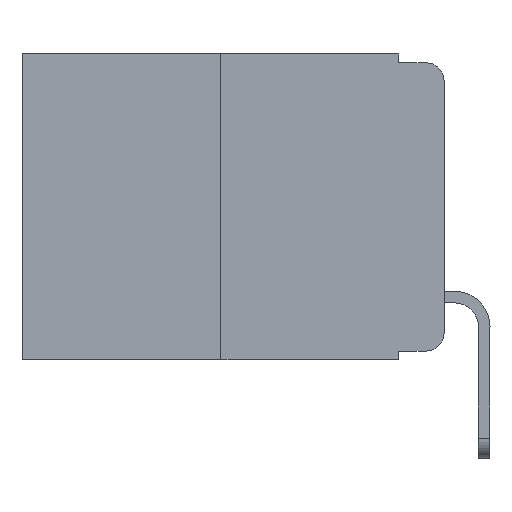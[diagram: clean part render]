
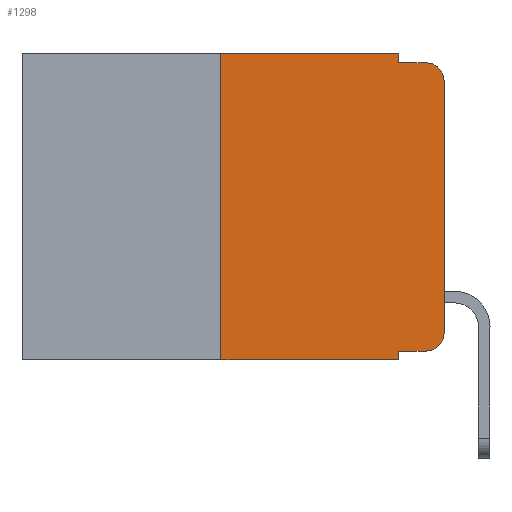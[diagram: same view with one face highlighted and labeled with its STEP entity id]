
A CAD part, left-side view. The second image highlights one B-rep face of the part: STEP entity #1298.
In plain terms, the highlighted planar face has unit normal (-1, 0, 0).
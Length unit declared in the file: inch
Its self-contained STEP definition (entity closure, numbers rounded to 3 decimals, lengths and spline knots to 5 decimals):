
#340 = VECTOR ( 'NONE', #1689, 39.37008 ) ;
#1086 = LINE ( 'NONE', #12152, #5563 ) ;
#1298 = ADVANCED_FACE ( 'NONE', ( #9779 ), #1872, .F. ) ;
#1528 = DIRECTION ( 'NONE',  ( -1., 0., 0. ) ) ;
#1554 = EDGE_CURVE ( 'NONE', #5342, #3291, #9195, .T. ) ;
#1689 = DIRECTION ( 'NONE',  ( 0., 0., 1. ) ) ;
#1758 = CARTESIAN_POINT ( 'NONE',  ( 0., 0.473, 0. ) ) ;
#1872 = PLANE ( 'NONE',  #3984 ) ;
#2071 = CARTESIAN_POINT ( 'NONE',  ( 0., 0., -0.03 ) ) ;
#2209 = LINE ( 'NONE', #12271, #6872 ) ;
#2765 = VERTEX_POINT ( 'NONE', #12022 ) ;
#2840 = VECTOR ( 'NONE', #3044, 39.37008 ) ;
#2890 = DIRECTION ( 'NONE',  ( 0., -1., 0. ) ) ;
#3044 = DIRECTION ( 'NONE',  ( 0., -1., 0. ) ) ;
#3227 = ORIENTED_EDGE ( 'NONE', *, *, #10108, .T. ) ;
#3291 = VERTEX_POINT ( 'NONE', #4524 ) ;
#3742 = DIRECTION ( 'NONE',  ( 0., 0., -1. ) ) ;
#3973 = ORIENTED_EDGE ( 'NONE', *, *, #14810, .F. ) ;
#3984 = AXIS2_PLACEMENT_3D ( 'NONE', #5562, #14246, #12817 ) ;
#4219 = EDGE_CURVE ( 'NONE', #8052, #2765, #6016, .T. ) ;
#4456 = EDGE_CURVE ( 'NONE', #11386, #15500, #11391, .T. ) ;
#4524 = CARTESIAN_POINT ( 'NONE',  ( 0., 0., -0.313 ) ) ;
#4906 = DIRECTION ( 'NONE',  ( 0., -1., 0. ) ) ;
#5342 = VERTEX_POINT ( 'NONE', #9818 ) ;
#5562 = CARTESIAN_POINT ( 'NONE',  ( 0., 0.473, 0. ) ) ;
#5563 = VECTOR ( 'NONE', #10189, 39.37008 ) ;
#5622 = EDGE_CURVE ( 'NONE', #15500, #10020, #9814, .T. ) ;
#6016 = CIRCLE ( 'NONE', #8974, 0.02 ) ;
#6192 = LINE ( 'NONE', #9088, #340 ) ;
#6570 = CARTESIAN_POINT ( 'NONE',  ( 0., 0.02, -0.03 ) ) ;
#6620 = ORIENTED_EDGE ( 'NONE', *, *, #5622, .F. ) ;
#6689 = AXIS2_PLACEMENT_3D ( 'NONE', #9867, #15855, #8411 ) ;
#6872 = VECTOR ( 'NONE', #4906, 39.37008 ) ;
#7347 = LINE ( 'NONE', #8785, #8878 ) ;
#7410 = CARTESIAN_POINT ( 'NONE',  ( 0., 0.25, 0. ) ) ;
#7444 = EDGE_CURVE ( 'NONE', #13667, #2765, #2209, .T. ) ;
#7505 = CARTESIAN_POINT ( 'NONE',  ( 0., 0.473, -0.343 ) ) ;
#7801 = DIRECTION ( 'NONE',  ( 0., 0., -1. ) ) ;
#7888 = EDGE_LOOP ( 'NONE', ( #14979, #8328, #7933, #9356, #6620, #11798, #13872, #3973, #3227, #8174 ) ) ;
#7933 = ORIENTED_EDGE ( 'NONE', *, *, #7444, .F. ) ;
#8052 = VERTEX_POINT ( 'NONE', #2071 ) ;
#8134 = CARTESIAN_POINT ( 'NONE',  ( 0., 0.25, 0. ) ) ;
#8174 = ORIENTED_EDGE ( 'NONE', *, *, #1554, .T. ) ;
#8244 = VECTOR ( 'NONE', #3742, 39.37008 ) ;
#8328 = ORIENTED_EDGE ( 'NONE', *, *, #4219, .T. ) ;
#8411 = DIRECTION ( 'NONE',  ( 0., 0., -1. ) ) ;
#8655 = VECTOR ( 'NONE', #11267, 39.37008 ) ;
#8785 = CARTESIAN_POINT ( 'NONE',  ( 0., 0.051, -0.333 ) ) ;
#8795 = CARTESIAN_POINT ( 'NONE',  ( 0., 0.051, -0.01 ) ) ;
#8878 = VECTOR ( 'NONE', #2890, 39.37008 ) ;
#8974 = AXIS2_PLACEMENT_3D ( 'NONE', #6570, #1528, #7801 ) ;
#9088 = CARTESIAN_POINT ( 'NONE',  ( 0., 0., 0. ) ) ;
#9195 = CIRCLE ( 'NONE', #6689, 0.02 ) ;
#9276 = VERTEX_POINT ( 'NONE', #11964 ) ;
#9356 = ORIENTED_EDGE ( 'NONE', *, *, #14271, .F. ) ;
#9587 = DIRECTION ( 'NONE',  ( 0., 0., 1. ) ) ;
#9779 = FACE_OUTER_BOUND ( 'NONE', #7888, .T. ) ;
#9814 = LINE ( 'NONE', #1758, #2840 ) ;
#9818 = CARTESIAN_POINT ( 'NONE',  ( 0., 0.02, -0.333 ) ) ;
#9867 = CARTESIAN_POINT ( 'NONE',  ( 0., 0.02, -0.313 ) ) ;
#10020 = VERTEX_POINT ( 'NONE', #15046 ) ;
#10108 = EDGE_CURVE ( 'NONE', #9276, #5342, #7347, .T. ) ;
#10189 = DIRECTION ( 'NONE',  ( 0., 0., -1. ) ) ;
#10801 = EDGE_CURVE ( 'NONE', #3291, #8052, #6192, .T. ) ;
#11267 = DIRECTION ( 'NONE',  ( 0., -1., 0. ) ) ;
#11386 = VERTEX_POINT ( 'NONE', #15391 ) ;
#11391 = LINE ( 'NONE', #8134, #12731 ) ;
#11572 = CARTESIAN_POINT ( 'NONE',  ( 0., 0.051, -0.343 ) ) ;
#11798 = ORIENTED_EDGE ( 'NONE', *, *, #4456, .F. ) ;
#11922 = VERTEX_POINT ( 'NONE', #11572 ) ;
#11964 = CARTESIAN_POINT ( 'NONE',  ( 0., 0.051, -0.333 ) ) ;
#12022 = CARTESIAN_POINT ( 'NONE',  ( 0., 0.02, -0.01 ) ) ;
#12152 = CARTESIAN_POINT ( 'NONE',  ( 0., 0.051, 0. ) ) ;
#12271 = CARTESIAN_POINT ( 'NONE',  ( 0., 0.051, -0.01 ) ) ;
#12731 = VECTOR ( 'NONE', #9587, 39.37008 ) ;
#12817 = DIRECTION ( 'NONE',  ( 0., 0., -1. ) ) ;
#12846 = LINE ( 'NONE', #14972, #8244 ) ;
#13112 = LINE ( 'NONE', #7505, #8655 ) ;
#13578 = EDGE_CURVE ( 'NONE', #11386, #11922, #13112, .T. ) ;
#13667 = VERTEX_POINT ( 'NONE', #8795 ) ;
#13872 = ORIENTED_EDGE ( 'NONE', *, *, #13578, .T. ) ;
#14246 = DIRECTION ( 'NONE',  ( 1., 0., 0. ) ) ;
#14271 = EDGE_CURVE ( 'NONE', #10020, #13667, #1086, .T. ) ;
#14810 = EDGE_CURVE ( 'NONE', #9276, #11922, #12846, .T. ) ;
#14972 = CARTESIAN_POINT ( 'NONE',  ( 0., 0.051, 0. ) ) ;
#14979 = ORIENTED_EDGE ( 'NONE', *, *, #10801, .T. ) ;
#15046 = CARTESIAN_POINT ( 'NONE',  ( 0., 0.051, 0. ) ) ;
#15391 = CARTESIAN_POINT ( 'NONE',  ( 0., 0.25, -0.343 ) ) ;
#15500 = VERTEX_POINT ( 'NONE', #7410 ) ;
#15855 = DIRECTION ( 'NONE',  ( -1., 0., 0. ) ) ;
